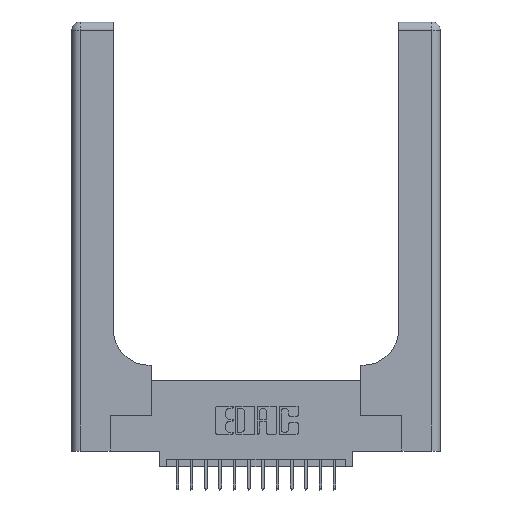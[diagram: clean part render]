
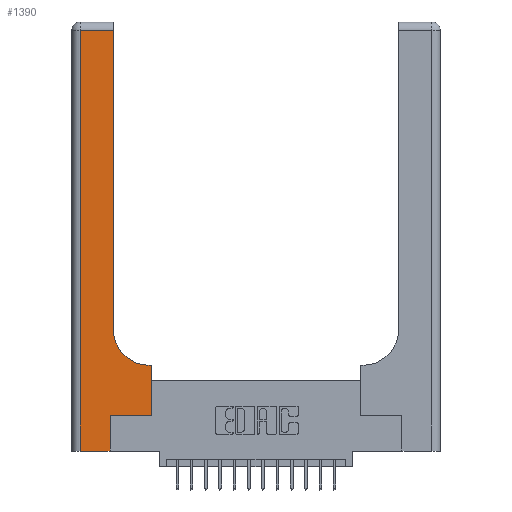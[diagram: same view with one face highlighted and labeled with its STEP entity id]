
A CAD part, top view. The second image highlights one B-rep face of the part: STEP entity #1390.
In plain terms, the highlighted planar face has unit normal (0, 0, 1).
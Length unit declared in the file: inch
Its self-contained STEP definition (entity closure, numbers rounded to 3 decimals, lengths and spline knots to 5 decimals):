
#709 = CARTESIAN_POINT ( 'NONE',  ( 0., 2.94, 0.37 ) ) ;
#711 = LINE ( 'NONE', #14209, #15401 ) ;
#848 = VECTOR ( 'NONE', #14700, 39.37008 ) ;
#942 = FACE_OUTER_BOUND ( 'NONE', #18507, .T. ) ;
#991 = LINE ( 'NONE', #1201, #4487 ) ;
#1097 = CARTESIAN_POINT ( 'NONE',  ( 0.5585, 0.25, 0.37 ) ) ;
#1159 = EDGE_CURVE ( 'NONE', #7497, #6468, #711, .T. ) ;
#1201 = CARTESIAN_POINT ( 'NONE',  ( 0.269, 0.25, 0.37 ) ) ;
#1390 = ADVANCED_FACE ( 'NONE', ( #942 ), #4610, .F. ) ;
#1741 = LINE ( 'NONE', #6088, #16361 ) ;
#2616 = DIRECTION ( 'NONE',  ( 0., 1., 0. ) ) ;
#3180 = AXIS2_PLACEMENT_3D ( 'NONE', #4070, #4007, #3982 ) ;
#3230 = LINE ( 'NONE', #709, #18213 ) ;
#3376 = EDGE_CURVE ( 'NONE', #11619, #4634, #7340, .T. ) ;
#3405 = CARTESIAN_POINT ( 'NONE',  ( 0.5585, 0.25, 0.37 ) ) ;
#3428 = VECTOR ( 'NONE', #6268, 39.37008 ) ;
#3709 = DIRECTION ( 'NONE',  ( -1., 0., 0. ) ) ;
#3845 = CARTESIAN_POINT ( 'NONE',  ( 0.269, 0., 0.37 ) ) ;
#3982 = DIRECTION ( 'NONE',  ( -1., 0., 0. ) ) ;
#4007 = DIRECTION ( 'NONE',  ( 0., 0., -1. ) ) ;
#4070 = CARTESIAN_POINT ( 'NONE',  ( 0., 3., 0.37 ) ) ;
#4482 = CARTESIAN_POINT ( 'NONE',  ( 0.06, 3., 0.37 ) ) ;
#4487 = VECTOR ( 'NONE', #18606, 39.37008 ) ;
#4610 = PLANE ( 'NONE',  #3180 ) ;
#4634 = VERTEX_POINT ( 'NONE', #14077 ) ;
#5138 = VERTEX_POINT ( 'NONE', #16409 ) ;
#5298 = ORIENTED_EDGE ( 'NONE', *, *, #15144, .T. ) ;
#5333 = DIRECTION ( 'NONE',  ( 1., 0., 0. ) ) ;
#6088 = CARTESIAN_POINT ( 'NONE',  ( 0.2915, 3., 0.37 ) ) ;
#6268 = DIRECTION ( 'NONE',  ( -1., 0., 0. ) ) ;
#6272 = EDGE_CURVE ( 'NONE', #6954, #7497, #12645, .T. ) ;
#6281 = CARTESIAN_POINT ( 'NONE',  ( 0.5415, 0.85, 0.37 ) ) ;
#6468 = VERTEX_POINT ( 'NONE', #10683 ) ;
#6746 = ORIENTED_EDGE ( 'NONE', *, *, #1159, .T. ) ;
#6954 = VERTEX_POINT ( 'NONE', #17687 ) ;
#7340 = LINE ( 'NONE', #7724, #3428 ) ;
#7381 = AXIS2_PLACEMENT_3D ( 'NONE', #6281, #16439, #7742 ) ;
#7455 = CIRCLE ( 'NONE', #7381, 0.25 ) ;
#7497 = VERTEX_POINT ( 'NONE', #13620 ) ;
#7604 = LINE ( 'NONE', #3845, #17330 ) ;
#7724 = CARTESIAN_POINT ( 'NONE',  ( 0.2915, 0.6, 0.37 ) ) ;
#7742 = DIRECTION ( 'NONE',  ( 1., 0., 0. ) ) ;
#7933 = ORIENTED_EDGE ( 'NONE', *, *, #12123, .T. ) ;
#8507 = EDGE_CURVE ( 'NONE', #13545, #5138, #1741, .T. ) ;
#9811 = CARTESIAN_POINT ( 'NONE',  ( 0.2915, 0.85, 0.37 ) ) ;
#10199 = ORIENTED_EDGE ( 'NONE', *, *, #8507, .T. ) ;
#10459 = VERTEX_POINT ( 'NONE', #3405 ) ;
#10683 = CARTESIAN_POINT ( 'NONE',  ( 0.269, 0., 0.37 ) ) ;
#11130 = ORIENTED_EDGE ( 'NONE', *, *, #12927, .T. ) ;
#11619 = VERTEX_POINT ( 'NONE', #13394 ) ;
#12123 = EDGE_CURVE ( 'NONE', #16767, #10459, #991, .T. ) ;
#12377 = ORIENTED_EDGE ( 'NONE', *, *, #6272, .T. ) ;
#12645 = LINE ( 'NONE', #4482, #848 ) ;
#12927 = EDGE_CURVE ( 'NONE', #4634, #13545, #7455, .T. ) ;
#13394 = CARTESIAN_POINT ( 'NONE',  ( 0.5585, 0.6, 0.37 ) ) ;
#13545 = VERTEX_POINT ( 'NONE', #9811 ) ;
#13585 = EDGE_CURVE ( 'NONE', #10459, #11619, #16733, .T. ) ;
#13620 = CARTESIAN_POINT ( 'NONE',  ( 0.06, 0., 0.37 ) ) ;
#14077 = CARTESIAN_POINT ( 'NONE',  ( 0.5415, 0.6, 0.37 ) ) ;
#14209 = CARTESIAN_POINT ( 'NONE',  ( 0., 0., 0.37 ) ) ;
#14700 = DIRECTION ( 'NONE',  ( 0., -1., 0. ) ) ;
#14761 = DIRECTION ( 'NONE',  ( 0., 1., 0. ) ) ;
#14994 = ORIENTED_EDGE ( 'NONE', *, *, #13585, .T. ) ;
#15073 = EDGE_CURVE ( 'NONE', #5138, #6954, #3230, .T. ) ;
#15144 = EDGE_CURVE ( 'NONE', #6468, #16767, #7604, .T. ) ;
#15401 = VECTOR ( 'NONE', #5333, 39.37008 ) ;
#16079 = ORIENTED_EDGE ( 'NONE', *, *, #3376, .T. ) ;
#16297 = VECTOR ( 'NONE', #2616, 39.37008 ) ;
#16361 = VECTOR ( 'NONE', #14761, 39.37008 ) ;
#16409 = CARTESIAN_POINT ( 'NONE',  ( 0.2915, 2.94, 0.37 ) ) ;
#16439 = DIRECTION ( 'NONE',  ( 0., 0., -1. ) ) ;
#16733 = LINE ( 'NONE', #1097, #16297 ) ;
#16739 = CARTESIAN_POINT ( 'NONE',  ( 0.269, 0.25, 0.37 ) ) ;
#16767 = VERTEX_POINT ( 'NONE', #16739 ) ;
#17330 = VECTOR ( 'NONE', #18332, 39.37008 ) ;
#17687 = CARTESIAN_POINT ( 'NONE',  ( 0.06, 2.94, 0.37 ) ) ;
#18213 = VECTOR ( 'NONE', #3709, 39.37008 ) ;
#18305 = ORIENTED_EDGE ( 'NONE', *, *, #15073, .T. ) ;
#18332 = DIRECTION ( 'NONE',  ( 0., 1., 0. ) ) ;
#18507 = EDGE_LOOP ( 'NONE', ( #10199, #18305, #12377, #6746, #5298, #7933, #14994, #16079, #11130 ) ) ;
#18606 = DIRECTION ( 'NONE',  ( 1., 0., 0. ) ) ;
